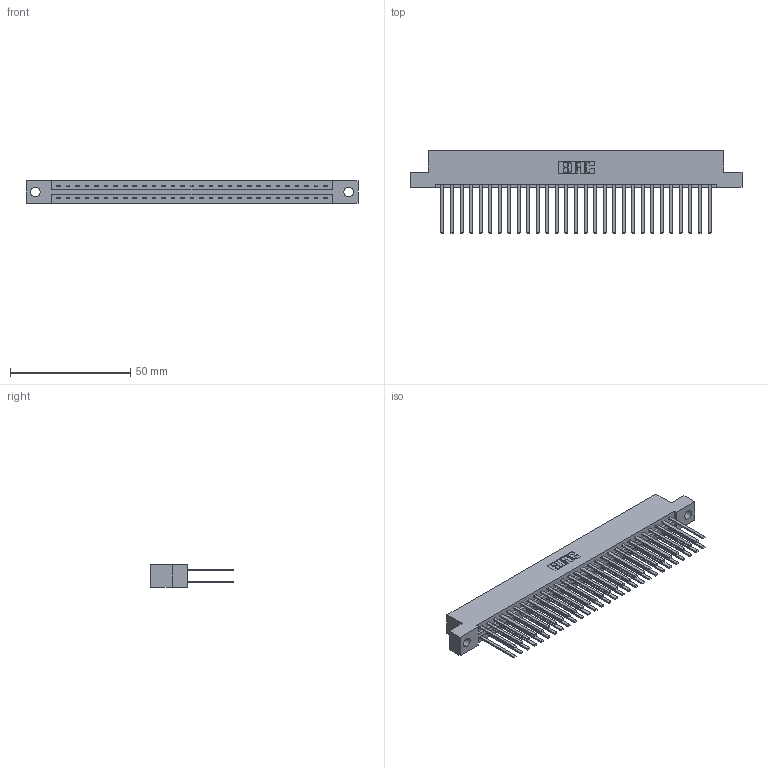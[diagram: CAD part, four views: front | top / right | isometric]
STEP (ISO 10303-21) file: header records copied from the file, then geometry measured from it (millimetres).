
FILE_DESCRIPTION (( 'STEP AP203' ), '1' );
FILE_NAME ('337-058-544-204.STEP', '2018-08-10T05:44:09', ( '' ), ( '' ), 'SwSTEP 2.0', 'SolidWorks 2016', '' );
FILE_SCHEMA (( 'CONFIG_CONTROL_DESIGN' ));
Length unit declared in the file: inch
Products named in the file (3): 337 Part_Flush Mounting Lugs - 0.156 Dia-TH; 345-292-001_345-293-144; 337-058-544-204
Assembly tree (59 placements, depth 2):
  337-058-544-204
    337 Part_Flush Mounting Lugs - 0.156 Dia-TH
    345-292-001_345-293-144  x58
Bounding box: 137.92 x 34.3 x 9.4 mm (x, y, z)
Volume: 15087.5 mm3; surface area: 19383.6 mm2
Topology: 59 solids, 59 shells, 2898 faces, 8605 edges, 5658 vertices
Faces by surface type: plane 2042, cylinder 856
Entity records: 23985 total; most frequent: CARTESIAN_POINT 4050, ORIENTED_EDGE 3986, DIRECTION 3465, EDGE_CURVE 1993, VECTOR 1869, LINE 1869, VERTEX_POINT 1326, AXIS2_PLACEMENT_3D 798
